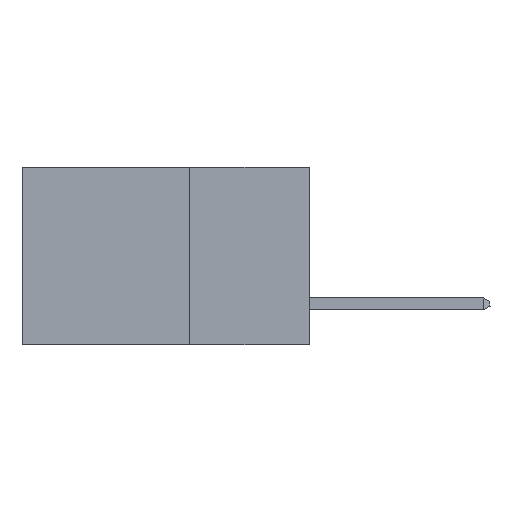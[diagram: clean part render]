
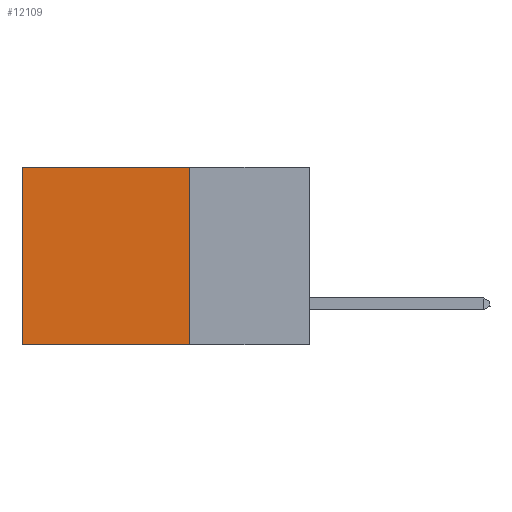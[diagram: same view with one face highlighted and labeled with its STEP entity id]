
A CAD part, left-side view. The second image highlights one B-rep face of the part: STEP entity #12109.
In plain terms, the highlighted planar face has unit normal (-1, 0, 0).
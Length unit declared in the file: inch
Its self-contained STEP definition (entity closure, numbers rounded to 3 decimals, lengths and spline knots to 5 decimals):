
#2816 = VECTOR ( 'NONE', #33878, 39.37008 ) ;
#7386 = DIRECTION ( 'NONE',  ( 0., 0., -1. ) ) ;
#8531 = DIRECTION ( 'NONE',  ( 0., 0., -1. ) ) ;
#9817 = EDGE_LOOP ( 'NONE', ( #17468, #22015, #43510, #20838 ) ) ;
#12109 = ADVANCED_FACE ( 'NONE', ( #19220 ), #43251, .F. ) ;
#16215 = CARTESIAN_POINT ( 'NONE',  ( 0.2875, 0.25, 0. ) ) ;
#16224 = VECTOR ( 'NONE', #18346, 39.37008 ) ;
#16377 = VECTOR ( 'NONE', #41248, 39.37008 ) ;
#17071 = CARTESIAN_POINT ( 'NONE',  ( 0.2875, 0.6, 0. ) ) ;
#17468 = ORIENTED_EDGE ( 'NONE', *, *, #38489, .T. ) ;
#17825 = LINE ( 'NONE', #28321, #35229 ) ;
#18346 = DIRECTION ( 'NONE',  ( 0., 1., 0. ) ) ;
#18607 = EDGE_CURVE ( 'NONE', #24858, #35561, #32264, .T. ) ;
#19107 = DIRECTION ( 'NONE',  ( 1., 0., 0. ) ) ;
#19220 = FACE_OUTER_BOUND ( 'NONE', #9817, .T. ) ;
#19626 = AXIS2_PLACEMENT_3D ( 'NONE', #25672, #19107, #8531 ) ;
#20838 = ORIENTED_EDGE ( 'NONE', *, *, #18607, .T. ) ;
#22015 = ORIENTED_EDGE ( 'NONE', *, *, #32533, .F. ) ;
#23912 = EDGE_CURVE ( 'NONE', #24858, #41812, #17825, .T. ) ;
#24858 = VERTEX_POINT ( 'NONE', #26564 ) ;
#25672 = CARTESIAN_POINT ( 'NONE',  ( 0.2875, 0.25, 0. ) ) ;
#25996 = LINE ( 'NONE', #42510, #16224 ) ;
#26564 = CARTESIAN_POINT ( 'NONE',  ( 0.2875, 0.25, 0. ) ) ;
#27667 = CARTESIAN_POINT ( 'NONE',  ( 0.2875, 0.6, -0.37 ) ) ;
#27835 = LINE ( 'NONE', #17071, #16377 ) ;
#28123 = CARTESIAN_POINT ( 'NONE',  ( 0.2875, 0.6, 0. ) ) ;
#28321 = CARTESIAN_POINT ( 'NONE',  ( 0.2875, 0.25, 0. ) ) ;
#32264 = LINE ( 'NONE', #16215, #2816 ) ;
#32533 = EDGE_CURVE ( 'NONE', #41812, #33625, #25996, .T. ) ;
#33625 = VERTEX_POINT ( 'NONE', #27667 ) ;
#33878 = DIRECTION ( 'NONE',  ( 0., 1., 0. ) ) ;
#35229 = VECTOR ( 'NONE', #7386, 39.37008 ) ;
#35561 = VERTEX_POINT ( 'NONE', #28123 ) ;
#35957 = CARTESIAN_POINT ( 'NONE',  ( 0.2875, 0.25, -0.37 ) ) ;
#38489 = EDGE_CURVE ( 'NONE', #35561, #33625, #27835, .T. ) ;
#41248 = DIRECTION ( 'NONE',  ( 0., 0., -1. ) ) ;
#41812 = VERTEX_POINT ( 'NONE', #35957 ) ;
#42510 = CARTESIAN_POINT ( 'NONE',  ( 0.2875, 0.25, -0.37 ) ) ;
#43251 = PLANE ( 'NONE',  #19626 ) ;
#43510 = ORIENTED_EDGE ( 'NONE', *, *, #23912, .F. ) ;
